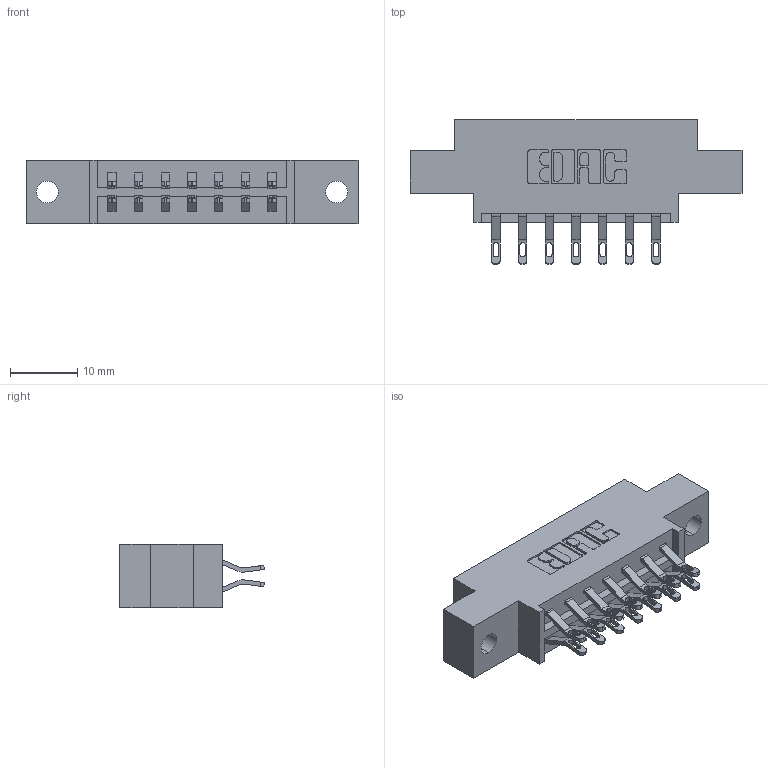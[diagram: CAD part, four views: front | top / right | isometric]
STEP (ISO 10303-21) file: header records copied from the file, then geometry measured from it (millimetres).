
FILE_DESCRIPTION (( 'STEP AP203' ), '1' );
FILE_NAME ('833-014-555-802.STEP', '2020-05-31T14:38:10', ( '' ), ( '' ), 'SwSTEP 2.0', 'SolidWorks 2020', '' );
FILE_SCHEMA (( 'CONFIG_CONTROL_DESIGN' ));
Length unit declared in the file: inch
Products named in the file (3): 345-292-001_555 Tail; 833-014-555-802; 833 Part_Offset - .128 Dia
Assembly tree (15 placements, depth 2):
  833-014-555-802
    833 Part_Offset - .128 Dia
    345-292-001_555 Tail  x14
Bounding box: 49.28 x 21.47 x 9.4 mm (x, y, z)
Volume: 4479.6 mm3; surface area: 5019.3 mm2
Topology: 15 solids, 15 shells, 930 faces, 2885 edges, 1922 vertices
Faces by surface type: plane 550, cylinder 380
Entity records: 9491 total; most frequent: CARTESIAN_POINT 1652, ORIENTED_EDGE 1558, DIRECTION 1443, EDGE_CURVE 779, LINE 631, VECTOR 631, VERTEX_POINT 518, AXIS2_PLACEMENT_3D 406
